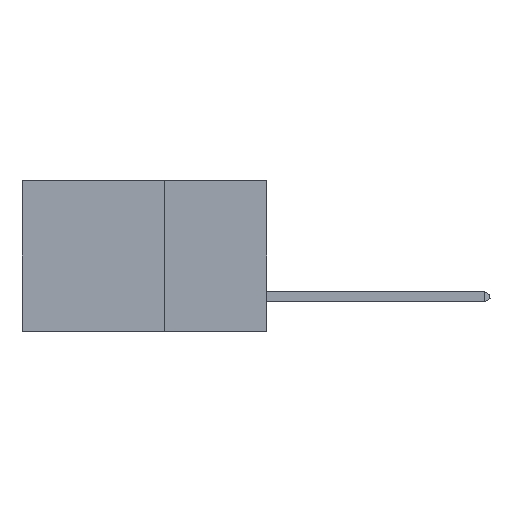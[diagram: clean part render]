
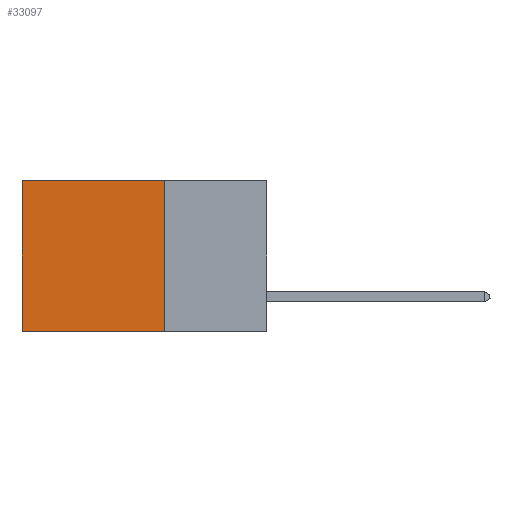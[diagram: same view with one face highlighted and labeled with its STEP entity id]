
A CAD part, left-side view. The second image highlights one B-rep face of the part: STEP entity #33097.
In plain terms, the highlighted planar face has unit normal (-1, 0, 0).
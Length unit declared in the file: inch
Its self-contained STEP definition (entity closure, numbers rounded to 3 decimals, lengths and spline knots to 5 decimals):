
#200 = CARTESIAN_POINT ( 'NONE',  ( 0.2875, 0.6, 0. ) ) ;
#2416 = ORIENTED_EDGE ( 'NONE', *, *, #36502, .T. ) ;
#2656 = VERTEX_POINT ( 'NONE', #200 ) ;
#5171 = CARTESIAN_POINT ( 'NONE',  ( 0.2875, 0.6, 0. ) ) ;
#6146 = DIRECTION ( 'NONE',  ( 0., 0., -1. ) ) ;
#6359 = PLANE ( 'NONE',  #24932 ) ;
#6851 = CARTESIAN_POINT ( 'NONE',  ( 0.2875, 0.25, 0. ) ) ;
#6891 = DIRECTION ( 'NONE',  ( 0., 1., 0. ) ) ;
#7839 = ORIENTED_EDGE ( 'NONE', *, *, #30289, .T. ) ;
#9111 = CARTESIAN_POINT ( 'NONE',  ( 0.2875, 0.25, -0.37 ) ) ;
#9971 = DIRECTION ( 'NONE',  ( 0., 0., -1. ) ) ;
#10993 = VECTOR ( 'NONE', #6146, 39.37008 ) ;
#15326 = VECTOR ( 'NONE', #6891, 39.37008 ) ;
#15658 = EDGE_LOOP ( 'NONE', ( #7839, #35367, #44504, #2416 ) ) ;
#15974 = DIRECTION ( 'NONE',  ( 0., 0., -1. ) ) ;
#17741 = CARTESIAN_POINT ( 'NONE',  ( 0.2875, 0.25, -0.37 ) ) ;
#18857 = EDGE_CURVE ( 'NONE', #41951, #43605, #37130, .T. ) ;
#20007 = VECTOR ( 'NONE', #15974, 39.37008 ) ;
#22704 = LINE ( 'NONE', #38016, #10993 ) ;
#24932 = AXIS2_PLACEMENT_3D ( 'NONE', #41670, #31154, #9971 ) ;
#29476 = LINE ( 'NONE', #30143, #41309 ) ;
#30143 = CARTESIAN_POINT ( 'NONE',  ( 0.2875, 0.25, 0. ) ) ;
#30289 = EDGE_CURVE ( 'NONE', #2656, #43605, #39547, .T. ) ;
#30897 = FACE_OUTER_BOUND ( 'NONE', #15658, .T. ) ;
#31154 = DIRECTION ( 'NONE',  ( 1., 0., 0. ) ) ;
#33097 = ADVANCED_FACE ( 'NONE', ( #30897 ), #6359, .F. ) ;
#34086 = DIRECTION ( 'NONE',  ( 0., 1., 0. ) ) ;
#35367 = ORIENTED_EDGE ( 'NONE', *, *, #18857, .F. ) ;
#36502 = EDGE_CURVE ( 'NONE', #37586, #2656, #29476, .T. ) ;
#37130 = LINE ( 'NONE', #9111, #15326 ) ;
#37586 = VERTEX_POINT ( 'NONE', #6851 ) ;
#38016 = CARTESIAN_POINT ( 'NONE',  ( 0.2875, 0.25, 0. ) ) ;
#39547 = LINE ( 'NONE', #5171, #20007 ) ;
#41309 = VECTOR ( 'NONE', #34086, 39.37008 ) ;
#41528 = CARTESIAN_POINT ( 'NONE',  ( 0.2875, 0.6, -0.37 ) ) ;
#41670 = CARTESIAN_POINT ( 'NONE',  ( 0.2875, 0.25, 0. ) ) ;
#41951 = VERTEX_POINT ( 'NONE', #17741 ) ;
#42500 = EDGE_CURVE ( 'NONE', #37586, #41951, #22704, .T. ) ;
#43605 = VERTEX_POINT ( 'NONE', #41528 ) ;
#44504 = ORIENTED_EDGE ( 'NONE', *, *, #42500, .F. ) ;
